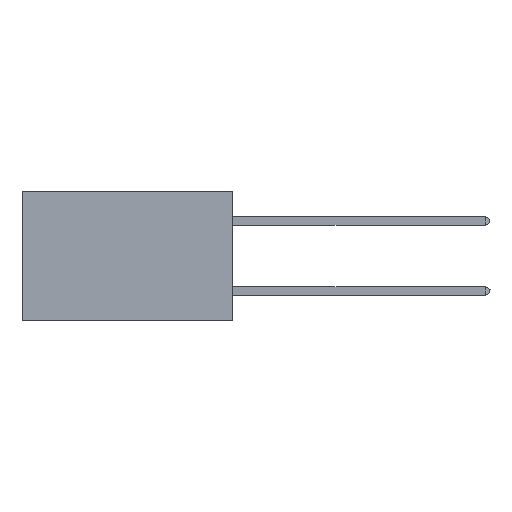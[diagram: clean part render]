
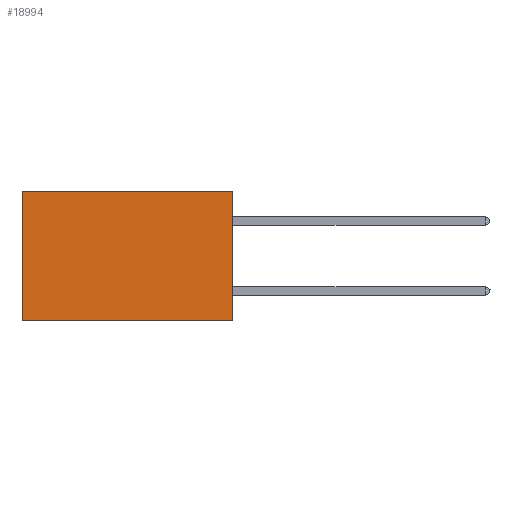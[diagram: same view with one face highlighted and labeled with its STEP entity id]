
A CAD part, left-side view. The second image highlights one B-rep face of the part: STEP entity #18994.
In plain terms, the highlighted planar face has unit normal (-1, 0, 0).
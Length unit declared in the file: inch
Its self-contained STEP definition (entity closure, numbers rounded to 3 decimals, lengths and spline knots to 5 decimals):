
#243 = ORIENTED_EDGE ( 'NONE', *, *, #7884, .T. ) ;
#825 = LINE ( 'NONE', #18369, #11692 ) ;
#1279 = CARTESIAN_POINT ( 'NONE',  ( 0.2875, 0., 0. ) ) ;
#2795 = CARTESIAN_POINT ( 'NONE',  ( 0.2875, 0., 0. ) ) ;
#4060 = VECTOR ( 'NONE', #15018, 39.37008 ) ;
#4899 = VECTOR ( 'NONE', #16005, 39.37008 ) ;
#6031 = LINE ( 'NONE', #19125, #4060 ) ;
#6132 = EDGE_LOOP ( 'NONE', ( #243, #21836, #22318, #25352 ) ) ;
#6937 = EDGE_CURVE ( 'NONE', #9284, #24672, #825, .T. ) ;
#7622 = CARTESIAN_POINT ( 'NONE',  ( 0.2875, 0., -0.37 ) ) ;
#7884 = EDGE_CURVE ( 'NONE', #24672, #15311, #6031, .T. ) ;
#7931 = DIRECTION ( 'NONE',  ( 0., 1., 0. ) ) ;
#9284 = VERTEX_POINT ( 'NONE', #1279 ) ;
#11260 = CARTESIAN_POINT ( 'NONE',  ( 0.2875, 0., -0.37 ) ) ;
#11692 = VECTOR ( 'NONE', #7931, 39.37008 ) ;
#12216 = DIRECTION ( 'NONE',  ( 0., 0., -1. ) ) ;
#13126 = EDGE_CURVE ( 'NONE', #9284, #25155, #16486, .T. ) ;
#13312 = DIRECTION ( 'NONE',  ( 1., 0., 0. ) ) ;
#13391 = DIRECTION ( 'NONE',  ( 0., 0., -1. ) ) ;
#14052 = CARTESIAN_POINT ( 'NONE',  ( 0.2875, 0., 0. ) ) ;
#15018 = DIRECTION ( 'NONE',  ( 0., 0., -1. ) ) ;
#15311 = VERTEX_POINT ( 'NONE', #25854 ) ;
#16005 = DIRECTION ( 'NONE',  ( 0., 1., 0. ) ) ;
#16486 = LINE ( 'NONE', #14052, #26389 ) ;
#18369 = CARTESIAN_POINT ( 'NONE',  ( 0.2875, 0., 0. ) ) ;
#18994 = ADVANCED_FACE ( 'NONE', ( #20251 ), #23887, .F. ) ;
#19125 = CARTESIAN_POINT ( 'NONE',  ( 0.2875, 0.6, 0. ) ) ;
#20251 = FACE_OUTER_BOUND ( 'NONE', #6132, .T. ) ;
#21836 = ORIENTED_EDGE ( 'NONE', *, *, #25403, .F. ) ;
#22239 = CARTESIAN_POINT ( 'NONE',  ( 0.2875, 0.6, 0. ) ) ;
#22318 = ORIENTED_EDGE ( 'NONE', *, *, #13126, .F. ) ;
#22775 = AXIS2_PLACEMENT_3D ( 'NONE', #2795, #13312, #13391 ) ;
#23887 = PLANE ( 'NONE',  #22775 ) ;
#24672 = VERTEX_POINT ( 'NONE', #22239 ) ;
#25155 = VERTEX_POINT ( 'NONE', #11260 ) ;
#25352 = ORIENTED_EDGE ( 'NONE', *, *, #6937, .T. ) ;
#25403 = EDGE_CURVE ( 'NONE', #25155, #15311, #25686, .T. ) ;
#25686 = LINE ( 'NONE', #7622, #4899 ) ;
#25854 = CARTESIAN_POINT ( 'NONE',  ( 0.2875, 0.6, -0.37 ) ) ;
#26389 = VECTOR ( 'NONE', #12216, 39.37008 ) ;
